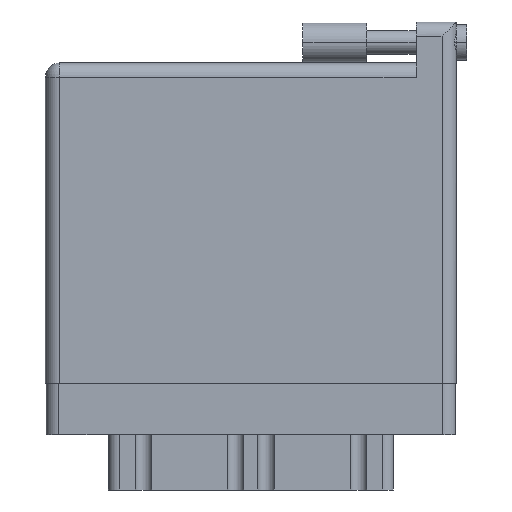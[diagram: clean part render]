
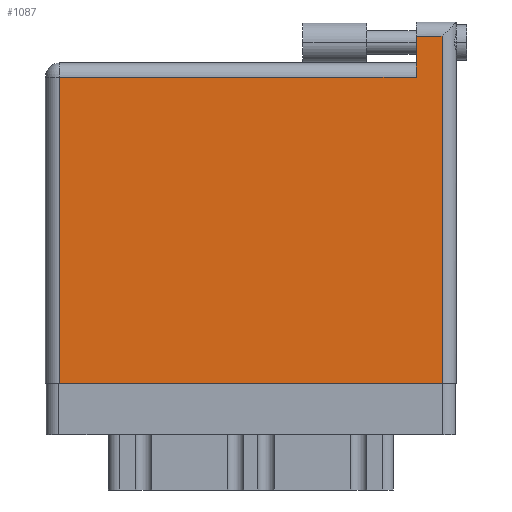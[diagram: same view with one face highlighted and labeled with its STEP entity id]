
A CAD part, front view. The second image highlights one B-rep face of the part: STEP entity #1087.
In plain terms, the highlighted face is planar.
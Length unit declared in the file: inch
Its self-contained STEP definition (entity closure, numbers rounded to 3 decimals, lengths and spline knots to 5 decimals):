
#411 = EDGE_CURVE ( 'NONE', #32409, #3987, #27725, .T. ) ;
#646 = VECTOR ( 'NONE', #6641, 39.37008 ) ;
#859 = AXIS2_PLACEMENT_3D ( 'NONE', #15627, #23817, #21391 ) ;
#1087 = ADVANCED_FACE ( 'NONE', ( #29230 ), #2238, .F. ) ;
#1317 = CARTESIAN_POINT ( 'NONE',  ( 1.811, 1.496, 0. ) ) ;
#1549 = VECTOR ( 'NONE', #24037, 39.37008 ) ;
#2238 = PLANE ( 'NONE',  #859 ) ;
#2244 = ORIENTED_EDGE ( 'NONE', *, *, #13171, .T. ) ;
#3007 = EDGE_CURVE ( 'NONE', #3987, #6082, #29279, .T. ) ;
#3871 = DIRECTION ( 'NONE',  ( 0., -1., 0. ) ) ;
#3987 = VERTEX_POINT ( 'NONE', #1317 ) ;
#4953 = LINE ( 'NONE', #15723, #11955 ) ;
#5606 = EDGE_CURVE ( 'NONE', #18057, #32409, #17241, .T. ) ;
#5711 = ORIENTED_EDGE ( 'NONE', *, *, #27977, .T. ) ;
#6082 = VERTEX_POINT ( 'NONE', #9215 ) ;
#6372 = ORIENTED_EDGE ( 'NONE', *, *, #9780, .T. ) ;
#6641 = DIRECTION ( 'NONE',  ( -1., 0., 0. ) ) ;
#7363 = ORIENTED_EDGE ( 'NONE', *, *, #3007, .T. ) ;
#8736 = ORIENTED_EDGE ( 'NONE', *, *, #411, .T. ) ;
#9215 = CARTESIAN_POINT ( 'NONE',  ( 0.07, 1.496, 0. ) ) ;
#9465 = EDGE_LOOP ( 'NONE', ( #6372, #5711, #19182, #8736, #7363, #2244 ) ) ;
#9780 = EDGE_CURVE ( 'NONE', #24719, #10184, #4953, .T. ) ;
#10184 = VERTEX_POINT ( 'NONE', #28927 ) ;
#10580 = CARTESIAN_POINT ( 'NONE',  ( 1.811, 1.696, 0. ) ) ;
#11955 = VECTOR ( 'NONE', #20974, 39.37008 ) ;
#13171 = EDGE_CURVE ( 'NONE', #6082, #24719, #16000, .T. ) ;
#15627 = CARTESIAN_POINT ( 'NONE',  ( 0., 1.566, 0. ) ) ;
#15723 = CARTESIAN_POINT ( 'NONE',  ( 0., 0., 0. ) ) ;
#16000 = LINE ( 'NONE', #29585, #19650 ) ;
#17078 = CARTESIAN_POINT ( 'NONE',  ( 0., 1.696, 0. ) ) ;
#17241 = LINE ( 'NONE', #17078, #646 ) ;
#18057 = VERTEX_POINT ( 'NONE', #22326 ) ;
#19182 = ORIENTED_EDGE ( 'NONE', *, *, #5606, .T. ) ;
#19650 = VECTOR ( 'NONE', #24008, 39.37008 ) ;
#20974 = DIRECTION ( 'NONE',  ( 1., 0., 0. ) ) ;
#21366 = VECTOR ( 'NONE', #3871, 39.37008 ) ;
#21391 = DIRECTION ( 'NONE',  ( -1., 0., 0. ) ) ;
#21393 = CARTESIAN_POINT ( 'NONE',  ( 1.938, 1.766, 0. ) ) ;
#21440 = CARTESIAN_POINT ( 'NONE',  ( 0., 1.496, 0. ) ) ;
#22326 = CARTESIAN_POINT ( 'NONE',  ( 1.938, 1.696, 0. ) ) ;
#23817 = DIRECTION ( 'NONE',  ( 0., 0., -1. ) ) ;
#24008 = DIRECTION ( 'NONE',  ( 0., -1., 0. ) ) ;
#24037 = DIRECTION ( 'NONE',  ( -1., 0., 0. ) ) ;
#24719 = VERTEX_POINT ( 'NONE', #27379 ) ;
#26446 = LINE ( 'NONE', #21393, #33233 ) ;
#27379 = CARTESIAN_POINT ( 'NONE',  ( 0.07, 0., 0. ) ) ;
#27725 = LINE ( 'NONE', #29993, #21366 ) ;
#27977 = EDGE_CURVE ( 'NONE', #10184, #18057, #26446, .T. ) ;
#28927 = CARTESIAN_POINT ( 'NONE',  ( 1.938, 0., 0. ) ) ;
#29230 = FACE_OUTER_BOUND ( 'NONE', #9465, .T. ) ;
#29279 = LINE ( 'NONE', #21440, #1549 ) ;
#29585 = CARTESIAN_POINT ( 'NONE',  ( 0.07, 0., 0. ) ) ;
#29993 = CARTESIAN_POINT ( 'NONE',  ( 1.811, 1.766, 0. ) ) ;
#32409 = VERTEX_POINT ( 'NONE', #10580 ) ;
#33233 = VECTOR ( 'NONE', #34118, 39.37008 ) ;
#34118 = DIRECTION ( 'NONE',  ( 0., 1., 0. ) ) ;
